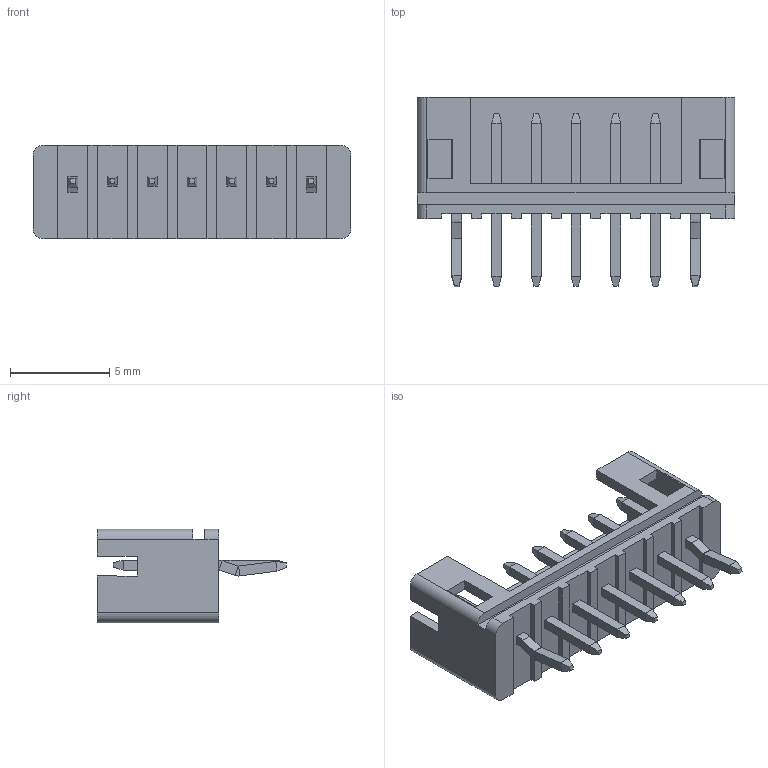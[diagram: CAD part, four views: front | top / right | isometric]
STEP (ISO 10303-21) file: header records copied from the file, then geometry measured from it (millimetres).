
FILE_DESCRIPTION (( 'STEP AP203' ), '1' );
FILE_NAME ('140-507-415-001.STEP', '2020-03-31T19:22:24', ( '' ), ( '' ), 'SwSTEP 2.0', 'SolidWorks 2016', '' );
FILE_SCHEMA (( 'CONFIG_CONTROL_DESIGN' ));
Length unit declared in the file: millimetre
Products named in the file (4): V Contact_Str; 140-507-415-001; V Contact_Kink; V Housing_507
Assembly tree (8 placements, depth 2):
  140-507-415-001
    V Housing_507
    V Contact_Kink  x2
    V Contact_Str  x5
Bounding box: 16 x 9.51 x 4.7 mm (x, y, z)
Volume: 175.8 mm3; surface area: 644.9 mm2
Topology: 8 solids, 8 shells, 224 faces, 550 edges, 340 vertices
Faces by surface type: plane 206, cylinder 16, bspline 2
Entity records: 4895 total; most frequent: CARTESIAN_POINT 800, ORIENTED_EDGE 750, DIRECTION 697, EDGE_CURVE 375, VECTOR 351, LINE 351, VERTEX_POINT 240, AXIS2_PLACEMENT_3D 173
